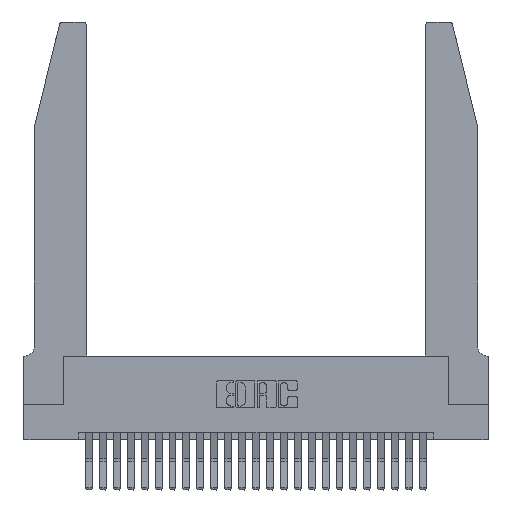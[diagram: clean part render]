
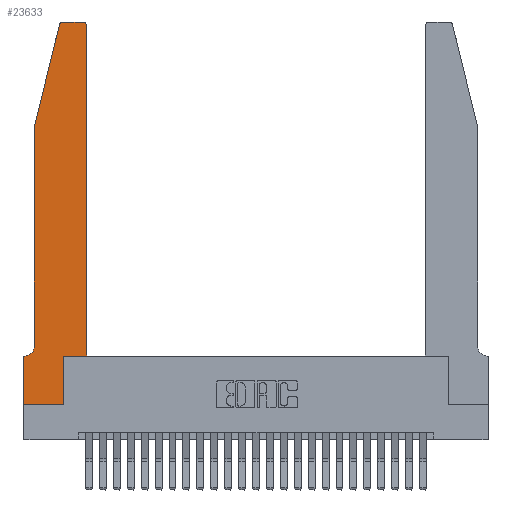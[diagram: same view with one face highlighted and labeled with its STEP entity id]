
A CAD part, top view. The second image highlights one B-rep face of the part: STEP entity #23633.
In plain terms, the highlighted planar face has unit normal (0, 0, 1).
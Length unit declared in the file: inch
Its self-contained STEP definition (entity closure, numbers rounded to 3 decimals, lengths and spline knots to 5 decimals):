
#630 = CARTESIAN_POINT ( 'NONE',  ( 0.0755, 2., 0.37 ) ) ;
#839 = CARTESIAN_POINT ( 'NONE',  ( 0.4505, 0.35, 0.37 ) ) ;
#1074 = AXIS2_PLACEMENT_3D ( 'NONE', #1878, #22345, #3790 ) ;
#1288 = CARTESIAN_POINT ( 'NONE',  ( 0.4505, 0.35, 0.37 ) ) ;
#1468 = VERTEX_POINT ( 'NONE', #19530 ) ;
#1663 = LINE ( 'NONE', #19169, #22302 ) ;
#1878 = CARTESIAN_POINT ( 'NONE',  ( 0.284, 2.72, 0.37 ) ) ;
#2130 = VERTEX_POINT ( 'NONE', #15373 ) ;
#2202 = EDGE_CURVE ( 'NONE', #21390, #2130, #13038, .T. ) ;
#2594 = EDGE_CURVE ( 'NONE', #1468, #25067, #4365, .T. ) ;
#2891 = CIRCLE ( 'NONE', #11906, 0.07 ) ;
#3105 = ORIENTED_EDGE ( 'NONE', *, *, #19553, .T. ) ;
#3307 = DIRECTION ( 'NONE',  ( 0., 0., 1. ) ) ;
#3422 = DIRECTION ( 'NONE',  ( -1., 0., 0. ) ) ;
#3790 = DIRECTION ( 'NONE',  ( 1., 0., 0. ) ) ;
#4365 = LINE ( 'NONE', #5928, #24996 ) ;
#4424 = EDGE_CURVE ( 'NONE', #17067, #17399, #1663, .T. ) ;
#4555 = ORIENTED_EDGE ( 'NONE', *, *, #16786, .T. ) ;
#4844 = ORIENTED_EDGE ( 'NONE', *, *, #2594, .T. ) ;
#5284 = DIRECTION ( 'NONE',  ( 0., 1., 0. ) ) ;
#5423 = EDGE_CURVE ( 'NONE', #15187, #7671, #19993, .T. ) ;
#5481 = CARTESIAN_POINT ( 'NONE',  ( 0.0755, 2., 0.37 ) ) ;
#5483 = PLANE ( 'NONE',  #5745 ) ;
#5530 = CARTESIAN_POINT ( 'NONE',  ( 0.0755, 0.35, 0.37 ) ) ;
#5643 = VECTOR ( 'NONE', #10921, 39.37008 ) ;
#5745 = AXIS2_PLACEMENT_3D ( 'NONE', #18055, #3307, #22121 ) ;
#5804 = VECTOR ( 'NONE', #5284, 39.37008 ) ;
#5928 = CARTESIAN_POINT ( 'NONE',  ( 0., 0., 0.37 ) ) ;
#6190 = DIRECTION ( 'NONE',  ( 0., 0., -1. ) ) ;
#6270 = CARTESIAN_POINT ( 'NONE',  ( 0.0055, 0.42, 0.37 ) ) ;
#6684 = CARTESIAN_POINT ( 'NONE',  ( 0.2865, 0., 0.37 ) ) ;
#6843 = ORIENTED_EDGE ( 'NONE', *, *, #9418, .T. ) ;
#7496 = CARTESIAN_POINT ( 'NONE',  ( 0.4205, 2.75, 0.37 ) ) ;
#7671 = VERTEX_POINT ( 'NONE', #21907 ) ;
#7672 = CARTESIAN_POINT ( 'NONE',  ( 0.2605, 2.75, 0.37 ) ) ;
#7929 = VERTEX_POINT ( 'NONE', #16229 ) ;
#8104 = CIRCLE ( 'NONE', #1074, 0.03 ) ;
#8228 = CARTESIAN_POINT ( 'NONE',  ( 0., 0., 0.37 ) ) ;
#8558 = DIRECTION ( 'NONE',  ( 0., 0., 1. ) ) ;
#8915 = CARTESIAN_POINT ( 'NONE',  ( 0.4505, 0.35, 0.37 ) ) ;
#9418 = EDGE_CURVE ( 'NONE', #25862, #15187, #9499, .T. ) ;
#9499 = CIRCLE ( 'NONE', #10171, 0.03 ) ;
#9737 = CARTESIAN_POINT ( 'NONE',  ( 0.2865, 0.35, 0.37 ) ) ;
#9743 = DIRECTION ( 'NONE',  ( -1., 0., 0. ) ) ;
#9969 = LINE ( 'NONE', #839, #5804 ) ;
#10048 = DIRECTION ( 'NONE',  ( 0., -1., 0. ) ) ;
#10171 = AXIS2_PLACEMENT_3D ( 'NONE', #18815, #8558, #21062 ) ;
#10921 = DIRECTION ( 'NONE',  ( -0.239, -0.971, 0. ) ) ;
#11226 = ORIENTED_EDGE ( 'NONE', *, *, #11891, .T. ) ;
#11367 = ORIENTED_EDGE ( 'NONE', *, *, #2202, .T. ) ;
#11814 = FACE_OUTER_BOUND ( 'NONE', #13936, .T. ) ;
#11865 = VECTOR ( 'NONE', #26114, 39.37008 ) ;
#11891 = EDGE_CURVE ( 'NONE', #7671, #7929, #8104, .T. ) ;
#11906 = AXIS2_PLACEMENT_3D ( 'NONE', #6270, #6190, #12241 ) ;
#12241 = DIRECTION ( 'NONE',  ( -1., 0., 0. ) ) ;
#13038 = LINE ( 'NONE', #5481, #19172 ) ;
#13049 = EDGE_CURVE ( 'NONE', #14944, #25862, #9969, .T. ) ;
#13736 = DIRECTION ( 'NONE',  ( 0., -1., 0. ) ) ;
#13881 = EDGE_CURVE ( 'NONE', #25984, #1468, #18937, .T. ) ;
#13936 = EDGE_LOOP ( 'NONE', ( #26599, #11226, #4555, #11367, #3105, #17506, #4844, #15647, #21337, #22587, #24527, #6843 ) ) ;
#14301 = VECTOR ( 'NONE', #18541, 39.37008 ) ;
#14497 = EDGE_CURVE ( 'NONE', #17399, #14944, #17609, .T. ) ;
#14944 = VERTEX_POINT ( 'NONE', #8915 ) ;
#15187 = VERTEX_POINT ( 'NONE', #7496 ) ;
#15373 = CARTESIAN_POINT ( 'NONE',  ( 0.0755, 0.42, 0.37 ) ) ;
#15647 = ORIENTED_EDGE ( 'NONE', *, *, #24428, .T. ) ;
#15763 = CARTESIAN_POINT ( 'NONE',  ( 0.0755, 2., 0.37 ) ) ;
#16229 = CARTESIAN_POINT ( 'NONE',  ( 0.25487, 2.72718, 0.37 ) ) ;
#16786 = EDGE_CURVE ( 'NONE', #7929, #21390, #18170, .T. ) ;
#17067 = VERTEX_POINT ( 'NONE', #6684 ) ;
#17386 = VECTOR ( 'NONE', #3422, 39.37008 ) ;
#17399 = VERTEX_POINT ( 'NONE', #9737 ) ;
#17506 = ORIENTED_EDGE ( 'NONE', *, *, #13881, .T. ) ;
#17609 = LINE ( 'NONE', #1288, #11865 ) ;
#18055 = CARTESIAN_POINT ( 'NONE',  ( 0., 0.35, 0.37 ) ) ;
#18170 = LINE ( 'NONE', #630, #5643 ) ;
#18541 = DIRECTION ( 'NONE',  ( 1., 0., 0. ) ) ;
#18605 = VECTOR ( 'NONE', #9743, 39.37008 ) ;
#18815 = CARTESIAN_POINT ( 'NONE',  ( 0.4205, 2.72, 0.37 ) ) ;
#18937 = LINE ( 'NONE', #5530, #18605 ) ;
#19169 = CARTESIAN_POINT ( 'NONE',  ( 0.2865, 0.35, 0.37 ) ) ;
#19172 = VECTOR ( 'NONE', #13736, 39.37008 ) ;
#19530 = CARTESIAN_POINT ( 'NONE',  ( 0., 0.35, 0.37 ) ) ;
#19553 = EDGE_CURVE ( 'NONE', #2130, #25984, #2891, .T. ) ;
#19993 = LINE ( 'NONE', #7672, #17386 ) ;
#20591 = CARTESIAN_POINT ( 'NONE',  ( 0., 0., 0.37 ) ) ;
#21062 = DIRECTION ( 'NONE',  ( 1., 0., 0. ) ) ;
#21337 = ORIENTED_EDGE ( 'NONE', *, *, #4424, .T. ) ;
#21390 = VERTEX_POINT ( 'NONE', #15763 ) ;
#21748 = LINE ( 'NONE', #8228, #14301 ) ;
#21907 = CARTESIAN_POINT ( 'NONE',  ( 0.284, 2.75, 0.37 ) ) ;
#22121 = DIRECTION ( 'NONE',  ( 1., 0., 0. ) ) ;
#22302 = VECTOR ( 'NONE', #25434, 39.37008 ) ;
#22345 = DIRECTION ( 'NONE',  ( 0., 0., 1. ) ) ;
#22587 = ORIENTED_EDGE ( 'NONE', *, *, #14497, .T. ) ;
#23611 = CARTESIAN_POINT ( 'NONE',  ( 0.4505, 2.72, 0.37 ) ) ;
#23633 = ADVANCED_FACE ( 'NONE', ( #11814 ), #5483, .T. ) ;
#24428 = EDGE_CURVE ( 'NONE', #25067, #17067, #21748, .T. ) ;
#24527 = ORIENTED_EDGE ( 'NONE', *, *, #13049, .T. ) ;
#24996 = VECTOR ( 'NONE', #10048, 39.37008 ) ;
#25067 = VERTEX_POINT ( 'NONE', #20591 ) ;
#25434 = DIRECTION ( 'NONE',  ( 0., 1., 0. ) ) ;
#25528 = CARTESIAN_POINT ( 'NONE',  ( 0.0055, 0.35, 0.37 ) ) ;
#25862 = VERTEX_POINT ( 'NONE', #23611 ) ;
#25984 = VERTEX_POINT ( 'NONE', #25528 ) ;
#26114 = DIRECTION ( 'NONE',  ( 1., 0., 0. ) ) ;
#26599 = ORIENTED_EDGE ( 'NONE', *, *, #5423, .T. ) ;
